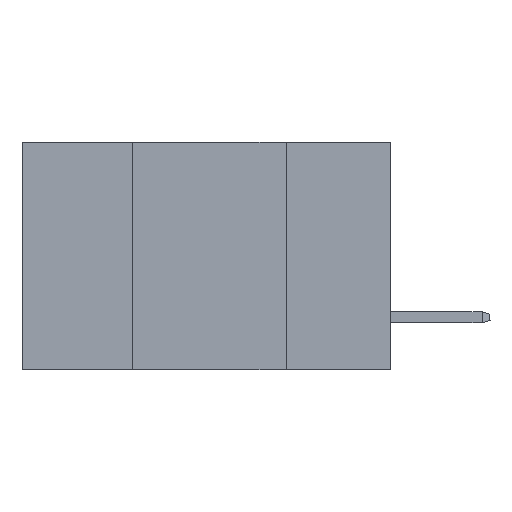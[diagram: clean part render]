
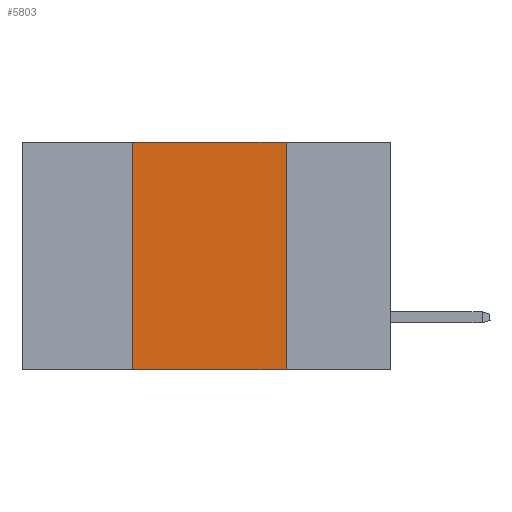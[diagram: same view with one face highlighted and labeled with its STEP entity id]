
A CAD part, left-side view. The second image highlights one B-rep face of the part: STEP entity #5803.
In plain terms, the highlighted planar face has unit normal (-1, 0, 0).
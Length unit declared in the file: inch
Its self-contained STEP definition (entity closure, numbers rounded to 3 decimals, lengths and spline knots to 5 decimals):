
#183 = CARTESIAN_POINT ( 'NONE',  ( 0., 0.42, 0. ) ) ;
#598 = CARTESIAN_POINT ( 'NONE',  ( 0., 0.6, 0. ) ) ;
#2092 = CARTESIAN_POINT ( 'NONE',  ( 0., 0.42, -0.37 ) ) ;
#2095 = ORIENTED_EDGE ( 'NONE', *, *, #12245, .F. ) ;
#2400 = CARTESIAN_POINT ( 'NONE',  ( 0., 0.17, -0.37 ) ) ;
#2401 = VERTEX_POINT ( 'NONE', #2400 ) ;
#2807 = FACE_OUTER_BOUND ( 'NONE', #9895, .T. ) ;
#2809 = VERTEX_POINT ( 'NONE', #2092 ) ;
#2813 = AXIS2_PLACEMENT_3D ( 'NONE', #9920, #7309, #4709 ) ;
#3508 = CARTESIAN_POINT ( 'NONE',  ( 0., 0.17, 0. ) ) ;
#3925 = LINE ( 'NONE', #3508, #7038 ) ;
#4709 = DIRECTION ( 'NONE',  ( 0., 0., -1. ) ) ;
#4725 = LINE ( 'NONE', #183, #5334 ) ;
#5151 = CARTESIAN_POINT ( 'NONE',  ( 0., 0.6, -0.37 ) ) ;
#5334 = VECTOR ( 'NONE', #9145, 39.37008 ) ;
#5535 = ORIENTED_EDGE ( 'NONE', *, *, #6142, .T. ) ;
#5803 = ADVANCED_FACE ( 'NONE', ( #2807 ), #16291, .F. ) ;
#6142 = EDGE_CURVE ( 'NONE', #2809, #2401, #7343, .T. ) ;
#7038 = VECTOR ( 'NONE', #9019, 39.37008 ) ;
#7309 = DIRECTION ( 'NONE',  ( 1., 0., 0. ) ) ;
#7343 = LINE ( 'NONE', #5151, #14882 ) ;
#8438 = LINE ( 'NONE', #598, #10470 ) ;
#9019 = DIRECTION ( 'NONE',  ( 0., 0., -1. ) ) ;
#9145 = DIRECTION ( 'NONE',  ( 0., 0., 1. ) ) ;
#9346 = EDGE_CURVE ( 'NONE', #13898, #2401, #3925, .T. ) ;
#9782 = DIRECTION ( 'NONE',  ( 0., -1., 0. ) ) ;
#9895 = EDGE_LOOP ( 'NONE', ( #15545, #2095, #16268, #5535 ) ) ;
#9920 = CARTESIAN_POINT ( 'NONE',  ( 0., 0.6, 0. ) ) ;
#10470 = VECTOR ( 'NONE', #9782, 39.37008 ) ;
#11968 = VERTEX_POINT ( 'NONE', #13977 ) ;
#12245 = EDGE_CURVE ( 'NONE', #11968, #13898, #8438, .T. ) ;
#13350 = EDGE_CURVE ( 'NONE', #2809, #11968, #4725, .T. ) ;
#13667 = CARTESIAN_POINT ( 'NONE',  ( 0., 0.17, 0. ) ) ;
#13898 = VERTEX_POINT ( 'NONE', #13667 ) ;
#13977 = CARTESIAN_POINT ( 'NONE',  ( 0., 0.42, 0. ) ) ;
#14159 = DIRECTION ( 'NONE',  ( 0., -1., 0. ) ) ;
#14882 = VECTOR ( 'NONE', #14159, 39.37008 ) ;
#15545 = ORIENTED_EDGE ( 'NONE', *, *, #9346, .F. ) ;
#16268 = ORIENTED_EDGE ( 'NONE', *, *, #13350, .F. ) ;
#16291 = PLANE ( 'NONE',  #2813 ) ;
